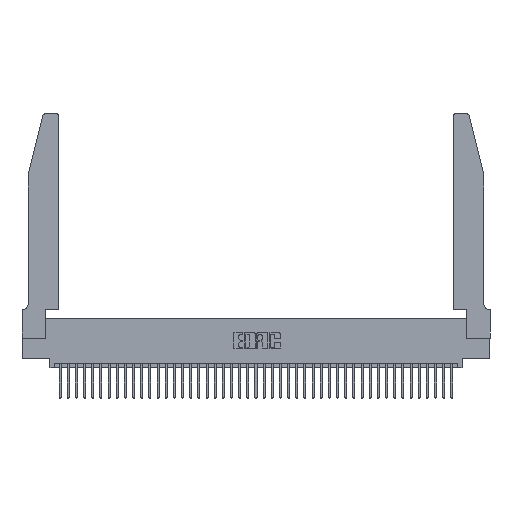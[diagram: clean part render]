
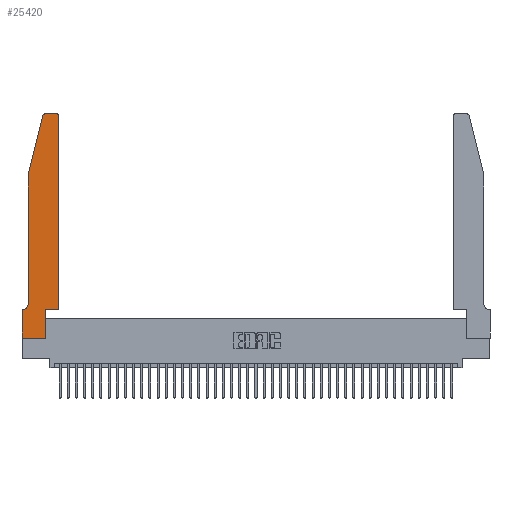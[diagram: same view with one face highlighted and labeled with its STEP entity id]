
A CAD part, top view. The second image highlights one B-rep face of the part: STEP entity #25420.
In plain terms, the highlighted planar face has unit normal (0, 0, 1).
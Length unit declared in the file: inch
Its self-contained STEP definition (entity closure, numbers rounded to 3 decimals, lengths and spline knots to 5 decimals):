
#291 = EDGE_LOOP ( 'NONE', ( #35121, #24193, #28256, #23066, #17933, #34539, #33917, #31023, #9689, #39583, #31954, #33468 ) ) ;
#712 = DIRECTION ( 'NONE',  ( 0., 0., 1. ) ) ;
#1015 = DIRECTION ( 'NONE',  ( 0., 0., 1. ) ) ;
#1570 = EDGE_CURVE ( 'NONE', #23457, #13736, #23081, .T. ) ;
#1774 = CARTESIAN_POINT ( 'NONE',  ( 0.2865, 0., 0.37 ) ) ;
#2845 = AXIS2_PLACEMENT_3D ( 'NONE', #10259, #712, #7409 ) ;
#3958 = VERTEX_POINT ( 'NONE', #1774 ) ;
#4297 = VECTOR ( 'NONE', #9082, 39.37008 ) ;
#4413 = EDGE_CURVE ( 'NONE', #35110, #14227, #27784, .T. ) ;
#4586 = CARTESIAN_POINT ( 'NONE',  ( 0.4505, 2.72, 0.37 ) ) ;
#4885 = DIRECTION ( 'NONE',  ( -0.239, -0.971, 0. ) ) ;
#5041 = DIRECTION ( 'NONE',  ( 0., 0., -1. ) ) ;
#5334 = DIRECTION ( 'NONE',  ( -1., 0., 0. ) ) ;
#5406 = AXIS2_PLACEMENT_3D ( 'NONE', #34974, #5041, #5334 ) ;
#6160 = DIRECTION ( 'NONE',  ( 0., -1., 0. ) ) ;
#6179 = LINE ( 'NONE', #41471, #33812 ) ;
#6191 = VERTEX_POINT ( 'NONE', #21646 ) ;
#7409 = DIRECTION ( 'NONE',  ( 1., 0., 0. ) ) ;
#7496 = EDGE_CURVE ( 'NONE', #12831, #25156, #30136, .T. ) ;
#7998 = EDGE_CURVE ( 'NONE', #25156, #6191, #14113, .T. ) ;
#8115 = CARTESIAN_POINT ( 'NONE',  ( 0., 0., 0.37 ) ) ;
#8448 = LINE ( 'NONE', #38582, #4297 ) ;
#8500 = CARTESIAN_POINT ( 'NONE',  ( 0.0755, 0.42, 0.37 ) ) ;
#8892 = CARTESIAN_POINT ( 'NONE',  ( 0.25487, 2.72718, 0.37 ) ) ;
#9082 = DIRECTION ( 'NONE',  ( 0., 1., 0. ) ) ;
#9689 = ORIENTED_EDGE ( 'NONE', *, *, #23535, .T. ) ;
#10259 = CARTESIAN_POINT ( 'NONE',  ( 0.284, 2.72, 0.37 ) ) ;
#11643 = CARTESIAN_POINT ( 'NONE',  ( 0., 0., 0.37 ) ) ;
#11841 = PLANE ( 'NONE',  #13473 ) ;
#11937 = FACE_OUTER_BOUND ( 'NONE', #291, .T. ) ;
#11984 = DIRECTION ( 'NONE',  ( 0., -1., 0. ) ) ;
#12831 = VERTEX_POINT ( 'NONE', #8500 ) ;
#13280 = LINE ( 'NONE', #11643, #36873 ) ;
#13473 = AXIS2_PLACEMENT_3D ( 'NONE', #15258, #18166, #41199 ) ;
#13736 = VERTEX_POINT ( 'NONE', #25623 ) ;
#13822 = EDGE_CURVE ( 'NONE', #18519, #14651, #26837, .T. ) ;
#14113 = LINE ( 'NONE', #40983, #38759 ) ;
#14227 = VERTEX_POINT ( 'NONE', #30732 ) ;
#14310 = AXIS2_PLACEMENT_3D ( 'NONE', #37334, #1015, #14666 ) ;
#14651 = VERTEX_POINT ( 'NONE', #14843 ) ;
#14666 = DIRECTION ( 'NONE',  ( 1., 0., 0. ) ) ;
#14843 = CARTESIAN_POINT ( 'NONE',  ( 0.0755, 2., 0.37 ) ) ;
#15258 = CARTESIAN_POINT ( 'NONE',  ( 0., 0.35, 0.37 ) ) ;
#16936 = VERTEX_POINT ( 'NONE', #38001 ) ;
#17705 = LINE ( 'NONE', #27639, #38751 ) ;
#17933 = ORIENTED_EDGE ( 'NONE', *, *, #7496, .T. ) ;
#18166 = DIRECTION ( 'NONE',  ( 0., 0., 1. ) ) ;
#18500 = VECTOR ( 'NONE', #22995, 39.37008 ) ;
#18519 = VERTEX_POINT ( 'NONE', #8892 ) ;
#21646 = CARTESIAN_POINT ( 'NONE',  ( 0., 0.35, 0.37 ) ) ;
#22995 = DIRECTION ( 'NONE',  ( -1., 0., 0. ) ) ;
#23066 = ORIENTED_EDGE ( 'NONE', *, *, #36875, .T. ) ;
#23081 = LINE ( 'NONE', #29713, #25125 ) ;
#23457 = VERTEX_POINT ( 'NONE', #32237 ) ;
#23535 = EDGE_CURVE ( 'NONE', #3958, #23457, #17705, .T. ) ;
#24193 = ORIENTED_EDGE ( 'NONE', *, *, #26572, .T. ) ;
#24485 = DIRECTION ( 'NONE',  ( 0., 1., 0. ) ) ;
#25125 = VECTOR ( 'NONE', #39161, 39.37008 ) ;
#25156 = VERTEX_POINT ( 'NONE', #30795 ) ;
#25196 = VECTOR ( 'NONE', #6160, 39.37008 ) ;
#25420 = ADVANCED_FACE ( 'NONE', ( #11937 ), #11841, .T. ) ;
#25623 = CARTESIAN_POINT ( 'NONE',  ( 0.4505, 0.35, 0.37 ) ) ;
#26572 = EDGE_CURVE ( 'NONE', #16936, #18519, #39526, .T. ) ;
#26837 = LINE ( 'NONE', #27396, #37570 ) ;
#27396 = CARTESIAN_POINT ( 'NONE',  ( 0.0755, 2., 0.37 ) ) ;
#27564 = DIRECTION ( 'NONE',  ( 1., 0., 0. ) ) ;
#27639 = CARTESIAN_POINT ( 'NONE',  ( 0.2865, 0.35, 0.37 ) ) ;
#27784 = CIRCLE ( 'NONE', #14310, 0.03 ) ;
#28137 = DIRECTION ( 'NONE',  ( -1., 0., 0. ) ) ;
#28256 = ORIENTED_EDGE ( 'NONE', *, *, #13822, .T. ) ;
#29713 = CARTESIAN_POINT ( 'NONE',  ( 0.4505, 0.35, 0.37 ) ) ;
#30136 = CIRCLE ( 'NONE', #5406, 0.07 ) ;
#30732 = CARTESIAN_POINT ( 'NONE',  ( 0.4205, 2.75, 0.37 ) ) ;
#30795 = CARTESIAN_POINT ( 'NONE',  ( 0.0055, 0.35, 0.37 ) ) ;
#31023 = ORIENTED_EDGE ( 'NONE', *, *, #40768, .T. ) ;
#31852 = LINE ( 'NONE', #35209, #25196 ) ;
#31896 = EDGE_CURVE ( 'NONE', #13736, #35110, #8448, .T. ) ;
#31954 = ORIENTED_EDGE ( 'NONE', *, *, #31896, .T. ) ;
#32237 = CARTESIAN_POINT ( 'NONE',  ( 0.2865, 0.35, 0.37 ) ) ;
#33468 = ORIENTED_EDGE ( 'NONE', *, *, #4413, .T. ) ;
#33812 = VECTOR ( 'NONE', #11984, 39.37008 ) ;
#33917 = ORIENTED_EDGE ( 'NONE', *, *, #33940, .T. ) ;
#33940 = EDGE_CURVE ( 'NONE', #6191, #42016, #31852, .T. ) ;
#34539 = ORIENTED_EDGE ( 'NONE', *, *, #7998, .T. ) ;
#34974 = CARTESIAN_POINT ( 'NONE',  ( 0.0055, 0.42, 0.37 ) ) ;
#35110 = VERTEX_POINT ( 'NONE', #4586 ) ;
#35121 = ORIENTED_EDGE ( 'NONE', *, *, #39629, .T. ) ;
#35209 = CARTESIAN_POINT ( 'NONE',  ( 0., 0., 0.37 ) ) ;
#36873 = VECTOR ( 'NONE', #27564, 39.37008 ) ;
#36875 = EDGE_CURVE ( 'NONE', #14651, #12831, #6179, .T. ) ;
#37334 = CARTESIAN_POINT ( 'NONE',  ( 0.4205, 2.72, 0.37 ) ) ;
#37570 = VECTOR ( 'NONE', #4885, 39.37008 ) ;
#38001 = CARTESIAN_POINT ( 'NONE',  ( 0.284, 2.75, 0.37 ) ) ;
#38582 = CARTESIAN_POINT ( 'NONE',  ( 0.4505, 0.35, 0.37 ) ) ;
#38751 = VECTOR ( 'NONE', #24485, 39.37008 ) ;
#38759 = VECTOR ( 'NONE', #28137, 39.37008 ) ;
#39088 = LINE ( 'NONE', #42428, #18500 ) ;
#39161 = DIRECTION ( 'NONE',  ( 1., 0., 0. ) ) ;
#39526 = CIRCLE ( 'NONE', #2845, 0.03 ) ;
#39583 = ORIENTED_EDGE ( 'NONE', *, *, #1570, .T. ) ;
#39629 = EDGE_CURVE ( 'NONE', #14227, #16936, #39088, .T. ) ;
#40768 = EDGE_CURVE ( 'NONE', #42016, #3958, #13280, .T. ) ;
#40983 = CARTESIAN_POINT ( 'NONE',  ( 0.0755, 0.35, 0.37 ) ) ;
#41199 = DIRECTION ( 'NONE',  ( 1., 0., 0. ) ) ;
#41471 = CARTESIAN_POINT ( 'NONE',  ( 0.0755, 2., 0.37 ) ) ;
#42016 = VERTEX_POINT ( 'NONE', #8115 ) ;
#42428 = CARTESIAN_POINT ( 'NONE',  ( 0.2605, 2.75, 0.37 ) ) ;
